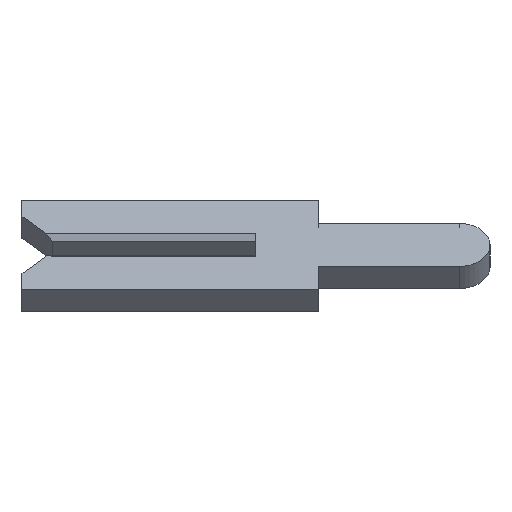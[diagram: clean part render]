
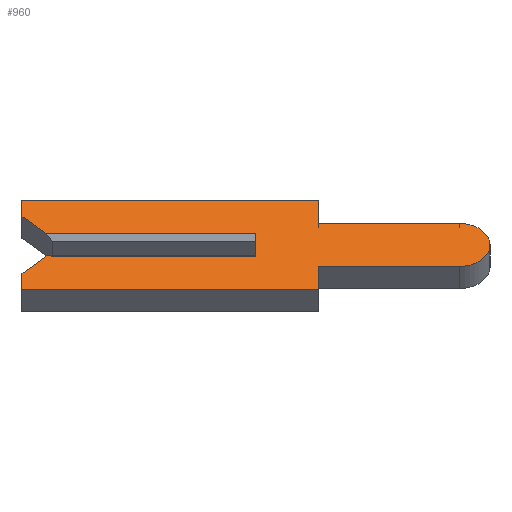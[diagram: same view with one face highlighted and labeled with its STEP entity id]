
A CAD part, left-side view. The second image highlights one B-rep face of the part: STEP entity #960.
In plain terms, the highlighted face is planar.
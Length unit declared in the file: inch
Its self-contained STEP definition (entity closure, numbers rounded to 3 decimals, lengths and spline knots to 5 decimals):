
#1 = VERTEX_POINT ( 'NONE', #185 ) ;
#16 = VERTEX_POINT ( 'NONE', #563 ) ;
#19 = LINE ( 'NONE', #170, #285 ) ;
#31 = DIRECTION ( 'NONE',  ( 0., 0., 1. ) ) ;
#40 = CARTESIAN_POINT ( 'NONE',  ( -0.01, -0.04, -0.04 ) ) ;
#44 = VERTEX_POINT ( 'NONE', #1149 ) ;
#46 = DIRECTION ( 'NONE',  ( 0., 0., 1. ) ) ;
#50 = LINE ( 'NONE', #353, #1013 ) ;
#56 = ORIENTED_EDGE ( 'NONE', *, *, #1096, .F. ) ;
#57 = DIRECTION ( 'NONE',  ( 0., 0., -1. ) ) ;
#59 = ORIENTED_EDGE ( 'NONE', *, *, #62, .F. ) ;
#62 = EDGE_CURVE ( 'NONE', #283, #664, #921, .T. ) ;
#67 = CARTESIAN_POINT ( 'NONE',  ( -0.01, 0.15, 0.04 ) ) ;
#72 = EDGE_CURVE ( 'NONE', #500, #345, #19, .T. ) ;
#76 = DIRECTION ( 'NONE',  ( 0., 0.707, 0.707 ) ) ;
#87 = VECTOR ( 'NONE', #1145, 39.37008 ) ;
#91 = CARTESIAN_POINT ( 'NONE',  ( -0.01, -0.04, -0.04 ) ) ;
#107 = LINE ( 'NONE', #1228, #323 ) ;
#116 = FACE_OUTER_BOUND ( 'NONE', #910, .T. ) ;
#121 = LINE ( 'NONE', #123, #892 ) ;
#123 = CARTESIAN_POINT ( 'NONE',  ( -0.01, -0.04, 0.04 ) ) ;
#136 = EDGE_CURVE ( 'NONE', #1025, #482, #1002, .T. ) ;
#137 = DIRECTION ( 'NONE',  ( 0., -1., 0. ) ) ;
#145 = VECTOR ( 'NONE', #641, 39.37008 ) ;
#156 = CARTESIAN_POINT ( 'NONE',  ( -0.01, -0.1305, 0. ) ) ;
#157 = ORIENTED_EDGE ( 'NONE', *, *, #621, .F. ) ;
#170 = CARTESIAN_POINT ( 'NONE',  ( -0.01, 0.1305, 0.0065 ) ) ;
#174 = VERTEX_POINT ( 'NONE', #286 ) ;
#180 = LINE ( 'NONE', #935, #87 ) ;
#185 = CARTESIAN_POINT ( 'NONE',  ( -0.01, -0.04, 0.0195 ) ) ;
#232 = VERTEX_POINT ( 'NONE', #866 ) ;
#236 = VECTOR ( 'NONE', #367, 39.37008 ) ;
#267 = DIRECTION ( 'NONE',  ( 0., -0.707, 0.707 ) ) ;
#268 = ORIENTED_EDGE ( 'NONE', *, *, #1072, .F. ) ;
#272 = ORIENTED_EDGE ( 'NONE', *, *, #1190, .T. ) ;
#281 = AXIS2_PLACEMENT_3D ( 'NONE', #1026, #1031, #446 ) ;
#283 = VERTEX_POINT ( 'NONE', #91 ) ;
#285 = VECTOR ( 'NONE', #76, 39.37008 ) ;
#286 = CARTESIAN_POINT ( 'NONE',  ( -0.01, 0.134, -0.01 ) ) ;
#323 = VECTOR ( 'NONE', #267, 39.37008 ) ;
#335 = VECTOR ( 'NONE', #57, 39.37008 ) ;
#339 = ORIENTED_EDGE ( 'NONE', *, *, #994, .F. ) ;
#345 = VERTEX_POINT ( 'NONE', #396 ) ;
#353 = CARTESIAN_POINT ( 'NONE',  ( -0.01, 0.15, 0.01 ) ) ;
#355 = DIRECTION ( 'NONE',  ( 0., 0., -1. ) ) ;
#367 = DIRECTION ( 'NONE',  ( 0., 0., 1. ) ) ;
#388 = ORIENTED_EDGE ( 'NONE', *, *, #831, .F. ) ;
#396 = CARTESIAN_POINT ( 'NONE',  ( -0.01, 0.15, 0.026 ) ) ;
#399 = ORIENTED_EDGE ( 'NONE', *, *, #835, .F. ) ;
#416 = CARTESIAN_POINT ( 'NONE',  ( -0.01, -0.1305, -0.0195 ) ) ;
#446 = DIRECTION ( 'NONE',  ( 0., 0., -1. ) ) ;
#479 = DIRECTION ( 'NONE',  ( 0., 1., 0. ) ) ;
#482 = VERTEX_POINT ( 'NONE', #859 ) ;
#500 = VERTEX_POINT ( 'NONE', #593 ) ;
#534 = EDGE_CURVE ( 'NONE', #345, #232, #991, .T. ) ;
#537 = LINE ( 'NONE', #40, #335 ) ;
#544 = ORIENTED_EDGE ( 'NONE', *, *, #136, .F. ) ;
#547 = DIRECTION ( 'NONE',  ( 1., 0., 0. ) ) ;
#554 = CARTESIAN_POINT ( 'NONE',  ( -0.01, 0., -0.01 ) ) ;
#559 = CARTESIAN_POINT ( 'NONE',  ( -0.01, -0.1305, 0.0195 ) ) ;
#563 = CARTESIAN_POINT ( 'NONE',  ( -0.01, -0.04, 0.04 ) ) ;
#581 = EDGE_CURVE ( 'NONE', #16, #1, #121, .T. ) ;
#593 = CARTESIAN_POINT ( 'NONE',  ( -0.01, 0.134, 0.01 ) ) ;
#596 = VECTOR ( 'NONE', #1136, 39.37008 ) ;
#621 = EDGE_CURVE ( 'NONE', #1209, #745, #1185, .T. ) ;
#633 = CARTESIAN_POINT ( 'NONE',  ( -0.01, -0.04, -0.0195 ) ) ;
#641 = DIRECTION ( 'NONE',  ( 0., -1., 0. ) ) ;
#664 = VERTEX_POINT ( 'NONE', #1100 ) ;
#671 = VECTOR ( 'NONE', #479, 39.37008 ) ;
#686 = AXIS2_PLACEMENT_3D ( 'NONE', #156, #547, #355 ) ;
#712 = CARTESIAN_POINT ( 'NONE',  ( -0.01, 0.15, -0.026 ) ) ;
#720 = CARTESIAN_POINT ( 'NONE',  ( -0.01, -0.04, 0.0195 ) ) ;
#725 = VECTOR ( 'NONE', #137, 39.37008 ) ;
#729 = ORIENTED_EDGE ( 'NONE', *, *, #534, .F. ) ;
#735 = VECTOR ( 'NONE', #31, 39.37008 ) ;
#745 = VERTEX_POINT ( 'NONE', #416 ) ;
#749 = DIRECTION ( 'NONE',  ( 0., -1., 0. ) ) ;
#751 = CARTESIAN_POINT ( 'NONE',  ( -0.01, 0.15, -0.04 ) ) ;
#826 = LINE ( 'NONE', #712, #1059 ) ;
#831 = EDGE_CURVE ( 'NONE', #924, #283, #537, .T. ) ;
#835 = EDGE_CURVE ( 'NONE', #664, #44, #826, .T. ) ;
#859 = CARTESIAN_POINT ( 'NONE',  ( -0.01, 0., 0.01 ) ) ;
#864 = ORIENTED_EDGE ( 'NONE', *, *, #581, .F. ) ;
#866 = CARTESIAN_POINT ( 'NONE',  ( -0.01, 0.15, 0.04 ) ) ;
#870 = LINE ( 'NONE', #67, #596 ) ;
#874 = ORIENTED_EDGE ( 'NONE', *, *, #919, .F. ) ;
#891 = DIRECTION ( 'NONE',  ( 0., 0., -1. ) ) ;
#892 = VECTOR ( 'NONE', #891, 39.37008 ) ;
#910 = EDGE_LOOP ( 'NONE', ( #272, #544, #56, #1018, #399, #59, #388, #268, #157, #874, #864, #339, #729, #1008 ) ) ;
#916 = LINE ( 'NONE', #927, #145 ) ;
#919 = EDGE_CURVE ( 'NONE', #1, #1209, #1107, .T. ) ;
#920 = PLANE ( 'NONE',  #281 ) ;
#921 = LINE ( 'NONE', #751, #671 ) ;
#924 = VERTEX_POINT ( 'NONE', #633 ) ;
#927 = CARTESIAN_POINT ( 'NONE',  ( -0.01, -0.1305, -0.01 ) ) ;
#935 = CARTESIAN_POINT ( 'NONE',  ( -0.01, -0.04, -0.0195 ) ) ;
#960 = ADVANCED_FACE ( 'NONE', ( #116 ), #920, .F. ) ;
#989 = CARTESIAN_POINT ( 'NONE',  ( -0.01, 0.15, 0.026 ) ) ;
#991 = LINE ( 'NONE', #989, #735 ) ;
#994 = EDGE_CURVE ( 'NONE', #232, #16, #870, .T. ) ;
#1002 = LINE ( 'NONE', #1052, #236 ) ;
#1008 = ORIENTED_EDGE ( 'NONE', *, *, #72, .F. ) ;
#1013 = VECTOR ( 'NONE', #749, 39.37008 ) ;
#1018 = ORIENTED_EDGE ( 'NONE', *, *, #1124, .F. ) ;
#1025 = VERTEX_POINT ( 'NONE', #554 ) ;
#1026 = CARTESIAN_POINT ( 'NONE',  ( -0.01, -0.1305, 0. ) ) ;
#1031 = DIRECTION ( 'NONE',  ( 1., 0., 0. ) ) ;
#1052 = CARTESIAN_POINT ( 'NONE',  ( -0.01, 0., 0.0065 ) ) ;
#1059 = VECTOR ( 'NONE', #46, 39.37008 ) ;
#1072 = EDGE_CURVE ( 'NONE', #745, #924, #180, .T. ) ;
#1096 = EDGE_CURVE ( 'NONE', #174, #1025, #916, .T. ) ;
#1100 = CARTESIAN_POINT ( 'NONE',  ( -0.01, 0.15, -0.04 ) ) ;
#1107 = LINE ( 'NONE', #720, #725 ) ;
#1124 = EDGE_CURVE ( 'NONE', #44, #174, #107, .T. ) ;
#1136 = DIRECTION ( 'NONE',  ( 0., -1., 0. ) ) ;
#1145 = DIRECTION ( 'NONE',  ( 0., 1., 0. ) ) ;
#1149 = CARTESIAN_POINT ( 'NONE',  ( -0.01, 0.15, -0.026 ) ) ;
#1185 = CIRCLE ( 'NONE', #686, 0.0195 ) ;
#1190 = EDGE_CURVE ( 'NONE', #500, #482, #50, .T. ) ;
#1209 = VERTEX_POINT ( 'NONE', #559 ) ;
#1228 = CARTESIAN_POINT ( 'NONE',  ( -0.01, 0.1305, -0.0065 ) ) ;
